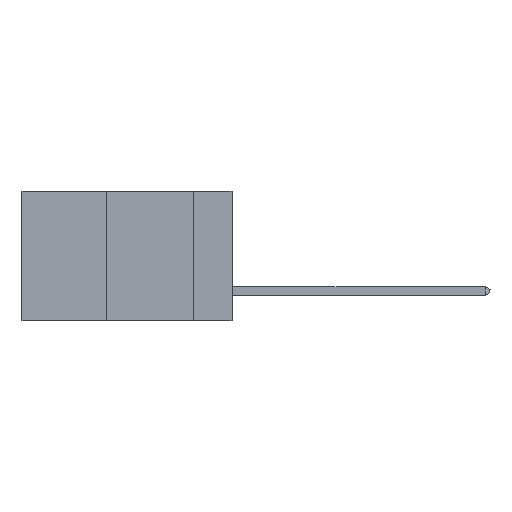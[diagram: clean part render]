
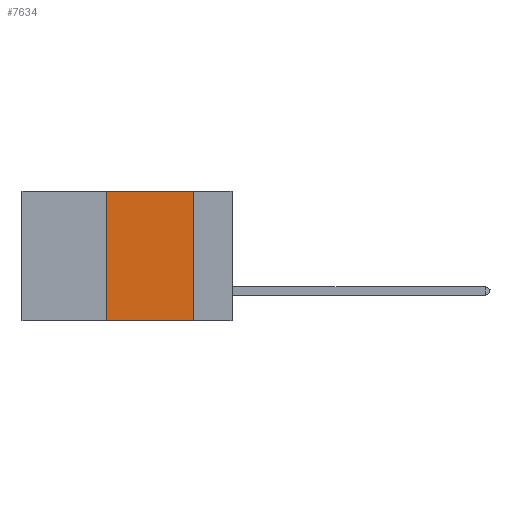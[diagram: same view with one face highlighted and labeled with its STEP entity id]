
A CAD part, left-side view. The second image highlights one B-rep face of the part: STEP entity #7634.
In plain terms, the highlighted planar face has unit normal (-1, 0, 0).
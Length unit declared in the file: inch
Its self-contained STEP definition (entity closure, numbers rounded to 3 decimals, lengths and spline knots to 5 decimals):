
#353 = LINE ( 'NONE', #12866, #4739 ) ;
#363 = ORIENTED_EDGE ( 'NONE', *, *, #3755, .F. ) ;
#557 = CARTESIAN_POINT ( 'NONE',  ( 0., 0.11, 0. ) ) ;
#2213 = LINE ( 'NONE', #17622, #7708 ) ;
#2694 = CARTESIAN_POINT ( 'NONE',  ( 0., 0.36, -0.37 ) ) ;
#3249 = DIRECTION ( 'NONE',  ( 0., -1., 0. ) ) ;
#3505 = CARTESIAN_POINT ( 'NONE',  ( 0., 0.6, -0.37 ) ) ;
#3755 = EDGE_CURVE ( 'NONE', #7632, #12290, #2213, .T. ) ;
#4546 = ORIENTED_EDGE ( 'NONE', *, *, #12628, .F. ) ;
#4739 = VECTOR ( 'NONE', #16022, 39.37008 ) ;
#5083 = CARTESIAN_POINT ( 'NONE',  ( 0., 0.36, 0. ) ) ;
#6247 = VECTOR ( 'NONE', #9676, 39.37008 ) ;
#6460 = PLANE ( 'NONE',  #13051 ) ;
#7632 = VERTEX_POINT ( 'NONE', #5083 ) ;
#7634 = ADVANCED_FACE ( 'NONE', ( #14682 ), #6460, .F. ) ;
#7708 = VECTOR ( 'NONE', #10333, 39.37008 ) ;
#7921 = DIRECTION ( 'NONE',  ( 1., 0., 0. ) ) ;
#8509 = EDGE_CURVE ( 'NONE', #11574, #18497, #10577, .T. ) ;
#9559 = DIRECTION ( 'NONE',  ( 0., 0., -1. ) ) ;
#9676 = DIRECTION ( 'NONE',  ( 0., 0., 1. ) ) ;
#10333 = DIRECTION ( 'NONE',  ( 0., -1., 0. ) ) ;
#10577 = LINE ( 'NONE', #3505, #18222 ) ;
#11574 = VERTEX_POINT ( 'NONE', #2694 ) ;
#12290 = VERTEX_POINT ( 'NONE', #557 ) ;
#12547 = CARTESIAN_POINT ( 'NONE',  ( 0., 0.11, -0.37 ) ) ;
#12628 = EDGE_CURVE ( 'NONE', #12290, #18497, #353, .T. ) ;
#12633 = CARTESIAN_POINT ( 'NONE',  ( 0., 0.36, 0. ) ) ;
#12866 = CARTESIAN_POINT ( 'NONE',  ( 0., 0.11, 0. ) ) ;
#13051 = AXIS2_PLACEMENT_3D ( 'NONE', #15537, #7921, #9559 ) ;
#14682 = FACE_OUTER_BOUND ( 'NONE', #16857, .T. ) ;
#15537 = CARTESIAN_POINT ( 'NONE',  ( 0., 0.6, 0. ) ) ;
#16022 = DIRECTION ( 'NONE',  ( 0., 0., -1. ) ) ;
#16857 = EDGE_LOOP ( 'NONE', ( #4546, #363, #18932, #18420 ) ) ;
#17622 = CARTESIAN_POINT ( 'NONE',  ( 0., 0.6, 0. ) ) ;
#18222 = VECTOR ( 'NONE', #3249, 39.37008 ) ;
#18420 = ORIENTED_EDGE ( 'NONE', *, *, #8509, .T. ) ;
#18497 = VERTEX_POINT ( 'NONE', #12547 ) ;
#18608 = LINE ( 'NONE', #12633, #6247 ) ;
#18932 = ORIENTED_EDGE ( 'NONE', *, *, #19079, .F. ) ;
#19079 = EDGE_CURVE ( 'NONE', #11574, #7632, #18608, .T. ) ;
